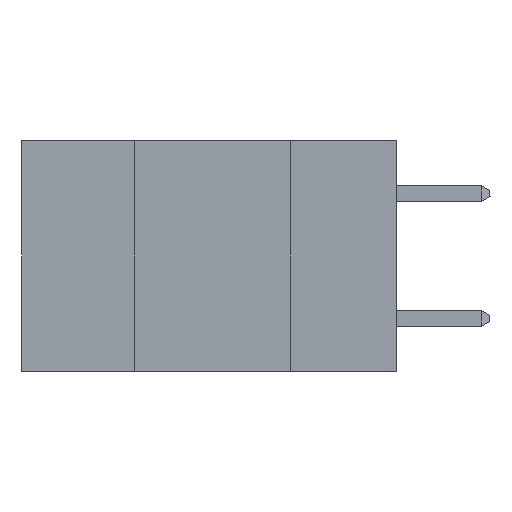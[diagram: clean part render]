
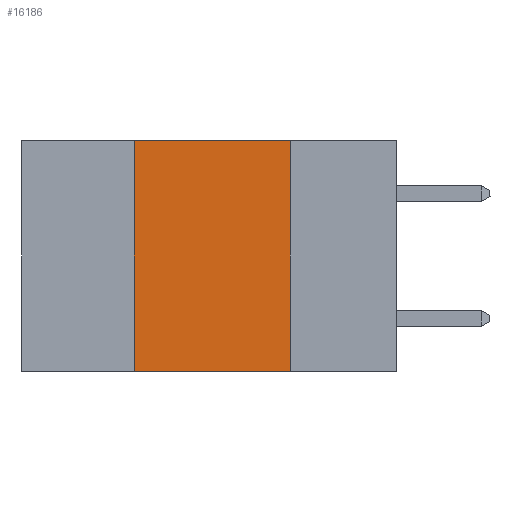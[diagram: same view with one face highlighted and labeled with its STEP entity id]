
A CAD part, left-side view. The second image highlights one B-rep face of the part: STEP entity #16186.
In plain terms, the highlighted planar face has unit normal (-1, 0, 0).
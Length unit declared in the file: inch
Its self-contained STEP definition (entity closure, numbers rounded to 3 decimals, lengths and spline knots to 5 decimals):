
#552 = DIRECTION ( 'NONE',  ( 1., 0., 0. ) ) ;
#1134 = LINE ( 'NONE', #1941, #13067 ) ;
#1162 = CARTESIAN_POINT ( 'NONE',  ( 0., 0.42, -0.37 ) ) ;
#1210 = LINE ( 'NONE', #15449, #6419 ) ;
#1564 = CARTESIAN_POINT ( 'NONE',  ( 0., 0.17, 0. ) ) ;
#1735 = ORIENTED_EDGE ( 'NONE', *, *, #16258, .F. ) ;
#1941 = CARTESIAN_POINT ( 'NONE',  ( 0., 0.6, 0. ) ) ;
#3233 = ORIENTED_EDGE ( 'NONE', *, *, #4166, .F. ) ;
#3431 = EDGE_LOOP ( 'NONE', ( #1735, #15576, #3233, #3610 ) ) ;
#3610 = ORIENTED_EDGE ( 'NONE', *, *, #8162, .T. ) ;
#4166 = EDGE_CURVE ( 'NONE', #13038, #10217, #5509, .T. ) ;
#4391 = CARTESIAN_POINT ( 'NONE',  ( 0., 0.42, 0. ) ) ;
#4438 = DIRECTION ( 'NONE',  ( 0., 0., -1. ) ) ;
#4823 = EDGE_CURVE ( 'NONE', #10217, #10882, #1134, .T. ) ;
#4895 = VERTEX_POINT ( 'NONE', #11287 ) ;
#5509 = LINE ( 'NONE', #12335, #16859 ) ;
#5534 = CARTESIAN_POINT ( 'NONE',  ( 0., 0.17, 0. ) ) ;
#6035 = DIRECTION ( 'NONE',  ( 0., -1., 0. ) ) ;
#6419 = VECTOR ( 'NONE', #7634, 39.37008 ) ;
#6654 = AXIS2_PLACEMENT_3D ( 'NONE', #8359, #552, #4438 ) ;
#6811 = FACE_OUTER_BOUND ( 'NONE', #3431, .T. ) ;
#7634 = DIRECTION ( 'NONE',  ( 0., -1., 0. ) ) ;
#8162 = EDGE_CURVE ( 'NONE', #13038, #4895, #1210, .T. ) ;
#8359 = CARTESIAN_POINT ( 'NONE',  ( 0., 0.6, 0. ) ) ;
#10217 = VERTEX_POINT ( 'NONE', #4391 ) ;
#10882 = VERTEX_POINT ( 'NONE', #5534 ) ;
#11136 = DIRECTION ( 'NONE',  ( 0., 0., 1. ) ) ;
#11287 = CARTESIAN_POINT ( 'NONE',  ( 0., 0.17, -0.37 ) ) ;
#11491 = VECTOR ( 'NONE', #12751, 39.37008 ) ;
#12335 = CARTESIAN_POINT ( 'NONE',  ( 0., 0.42, 0. ) ) ;
#12751 = DIRECTION ( 'NONE',  ( 0., 0., -1. ) ) ;
#13038 = VERTEX_POINT ( 'NONE', #1162 ) ;
#13067 = VECTOR ( 'NONE', #6035, 39.37008 ) ;
#15425 = LINE ( 'NONE', #1564, #11491 ) ;
#15449 = CARTESIAN_POINT ( 'NONE',  ( 0., 0.6, -0.37 ) ) ;
#15576 = ORIENTED_EDGE ( 'NONE', *, *, #4823, .F. ) ;
#16186 = ADVANCED_FACE ( 'NONE', ( #6811 ), #16280, .F. ) ;
#16258 = EDGE_CURVE ( 'NONE', #10882, #4895, #15425, .T. ) ;
#16280 = PLANE ( 'NONE',  #6654 ) ;
#16859 = VECTOR ( 'NONE', #11136, 39.37008 ) ;
